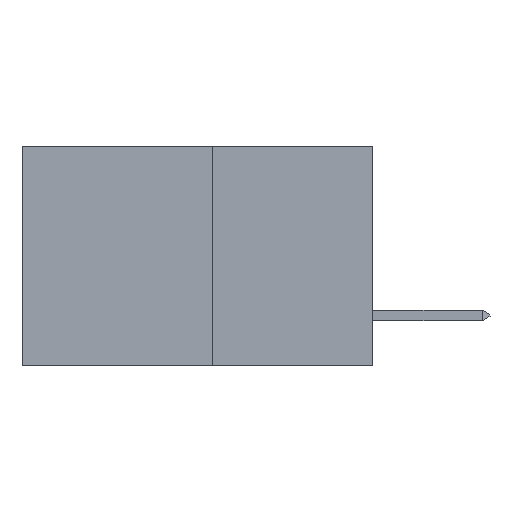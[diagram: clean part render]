
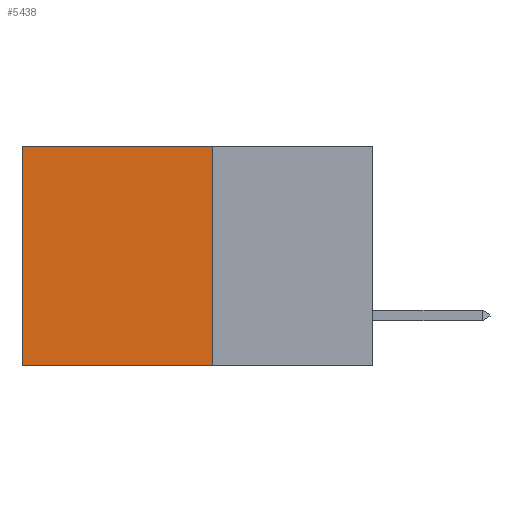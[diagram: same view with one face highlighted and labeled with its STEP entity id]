
A CAD part, left-side view. The second image highlights one B-rep face of the part: STEP entity #5438.
In plain terms, the highlighted planar face has unit normal (-1, 0, 0).
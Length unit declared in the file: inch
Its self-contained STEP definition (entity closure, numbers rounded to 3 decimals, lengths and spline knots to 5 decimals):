
#145 = VERTEX_POINT ( 'NONE', #7811 ) ;
#155 = CARTESIAN_POINT ( 'NONE',  ( 0.277, 0.27, -0.37 ) ) ;
#880 = LINE ( 'NONE', #8728, #5445 ) ;
#1300 = LINE ( 'NONE', #3070, #10267 ) ;
#1564 = VERTEX_POINT ( 'NONE', #10306 ) ;
#1617 = FACE_OUTER_BOUND ( 'NONE', #4287, .T. ) ;
#1703 = VECTOR ( 'NONE', #5612, 39.37008 ) ;
#3012 = VERTEX_POINT ( 'NONE', #9862 ) ;
#3070 = CARTESIAN_POINT ( 'NONE',  ( 0.277, 0.27, 0. ) ) ;
#3286 = DIRECTION ( 'NONE',  ( 0., 0., -1. ) ) ;
#4287 = EDGE_LOOP ( 'NONE', ( #6802, #4382, #6273, #5831 ) ) ;
#4382 = ORIENTED_EDGE ( 'NONE', *, *, #10832, .F. ) ;
#5137 = DIRECTION ( 'NONE',  ( 0., 1., 0. ) ) ;
#5299 = DIRECTION ( 'NONE',  ( 0., 0., -1. ) ) ;
#5438 = ADVANCED_FACE ( 'NONE', ( #1617 ), #7613, .F. ) ;
#5445 = VECTOR ( 'NONE', #5299, 39.37008 ) ;
#5612 = DIRECTION ( 'NONE',  ( 0., 0., -1. ) ) ;
#5831 = ORIENTED_EDGE ( 'NONE', *, *, #5931, .T. ) ;
#5931 = EDGE_CURVE ( 'NONE', #145, #3012, #1300, .T. ) ;
#5944 = CARTESIAN_POINT ( 'NONE',  ( 0.277, 0.27, -0.37 ) ) ;
#6273 = ORIENTED_EDGE ( 'NONE', *, *, #7790, .F. ) ;
#6443 = LINE ( 'NONE', #155, #1703 ) ;
#6802 = ORIENTED_EDGE ( 'NONE', *, *, #8858, .T. ) ;
#7613 = PLANE ( 'NONE',  #9323 ) ;
#7790 = EDGE_CURVE ( 'NONE', #145, #1564, #6443, .T. ) ;
#7811 = CARTESIAN_POINT ( 'NONE',  ( 0.277, 0.27, 0. ) ) ;
#8452 = LINE ( 'NONE', #10920, #10090 ) ;
#8509 = DIRECTION ( 'NONE',  ( 1., 0., 0. ) ) ;
#8728 = CARTESIAN_POINT ( 'NONE',  ( 0.277, 0.59, -0.37 ) ) ;
#8858 = EDGE_CURVE ( 'NONE', #3012, #9074, #880, .T. ) ;
#8969 = CARTESIAN_POINT ( 'NONE',  ( 0.277, 0.59, -0.37 ) ) ;
#9074 = VERTEX_POINT ( 'NONE', #8969 ) ;
#9323 = AXIS2_PLACEMENT_3D ( 'NONE', #5944, #8509, #3286 ) ;
#9862 = CARTESIAN_POINT ( 'NONE',  ( 0.277, 0.59, 0. ) ) ;
#10090 = VECTOR ( 'NONE', #5137, 39.37008 ) ;
#10267 = VECTOR ( 'NONE', #10729, 39.37008 ) ;
#10306 = CARTESIAN_POINT ( 'NONE',  ( 0.277, 0.27, -0.37 ) ) ;
#10729 = DIRECTION ( 'NONE',  ( 0., 1., 0. ) ) ;
#10832 = EDGE_CURVE ( 'NONE', #1564, #9074, #8452, .T. ) ;
#10920 = CARTESIAN_POINT ( 'NONE',  ( 0.277, 0.27, -0.37 ) ) ;
